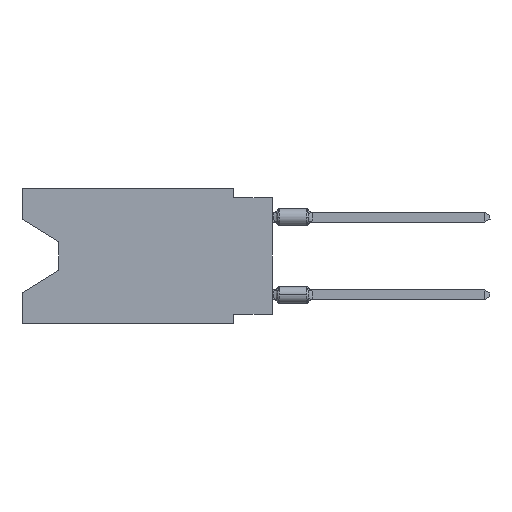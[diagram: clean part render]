
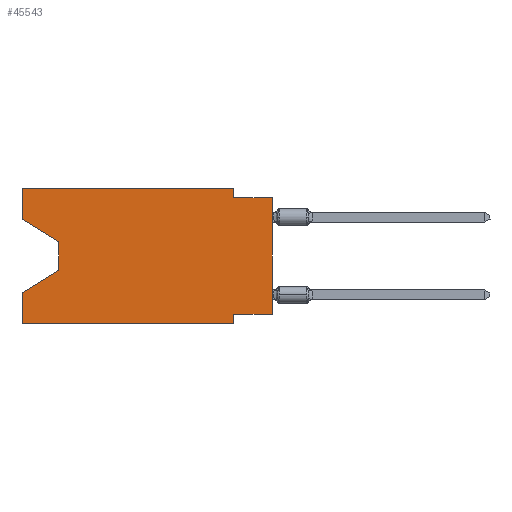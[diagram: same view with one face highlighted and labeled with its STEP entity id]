
A CAD part, left-side view. The second image highlights one B-rep face of the part: STEP entity #45543.
In plain terms, the highlighted planar face has unit normal (-1, 0, 0).
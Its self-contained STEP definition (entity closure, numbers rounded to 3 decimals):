
#326 = ORIENTED_EDGE ( 'NONE', *, *, #33293, .T. ) ;
#357 = DIRECTION ( 'NONE',  ( 0., -1., 0. ) ) ;
#640 = VECTOR ( 'NONE', #40639, 1000. ) ;
#901 = DIRECTION ( 'NONE',  ( 0., 0., -1. ) ) ;
#928 = EDGE_CURVE ( 'NONE', #18236, #33022, #54959, .T. ) ;
#1492 = CARTESIAN_POINT ( 'NONE',  ( 0., 0., -0.635 ) ) ;
#1679 = CARTESIAN_POINT ( 'NONE',  ( 0., 16.383, 0. ) ) ;
#2048 = VECTOR ( 'NONE', #901, 1000. ) ;
#2171 = LINE ( 'NONE', #29667, #26719 ) ;
#2493 = LINE ( 'NONE', #36974, #19120 ) ;
#5666 = CARTESIAN_POINT ( 'NONE',  ( 0., 13.97, -5.385 ) ) ;
#6044 = CARTESIAN_POINT ( 'NONE',  ( 0., 2.54, -8.89 ) ) ;
#7117 = LINE ( 'NONE', #29249, #27710 ) ;
#7543 = EDGE_CURVE ( 'NONE', #15446, #8250, #2493, .T. ) ;
#7650 = CARTESIAN_POINT ( 'NONE',  ( 0., 13.97, -3.505 ) ) ;
#8250 = VERTEX_POINT ( 'NONE', #22980 ) ;
#8898 = DIRECTION ( 'NONE',  ( 1., 0., 0. ) ) ;
#10454 = CARTESIAN_POINT ( 'NONE',  ( 0., 0., -8.255 ) ) ;
#10478 = ORIENTED_EDGE ( 'NONE', *, *, #29327, .T. ) ;
#11455 = LINE ( 'NONE', #28986, #30666 ) ;
#13536 = AXIS2_PLACEMENT_3D ( 'NONE', #30455, #8898, #48000 ) ;
#13838 = VERTEX_POINT ( 'NONE', #42373 ) ;
#15159 = DIRECTION ( 'NONE',  ( 0., 0., -1. ) ) ;
#15446 = VERTEX_POINT ( 'NONE', #5666 ) ;
#15514 = LINE ( 'NONE', #1492, #50405 ) ;
#17047 = CARTESIAN_POINT ( 'NONE',  ( 0., 16.383, -2.038 ) ) ;
#18236 = VERTEX_POINT ( 'NONE', #27883 ) ;
#19120 = VECTOR ( 'NONE', #33236, 1000. ) ;
#20636 = ORIENTED_EDGE ( 'NONE', *, *, #44938, .F. ) ;
#21025 = DIRECTION ( 'NONE',  ( 0., -1., 0. ) ) ;
#21209 = EDGE_CURVE ( 'NONE', #27404, #33022, #15514, .T. ) ;
#21676 = ORIENTED_EDGE ( 'NONE', *, *, #928, .T. ) ;
#22693 = VERTEX_POINT ( 'NONE', #22965 ) ;
#22965 = CARTESIAN_POINT ( 'NONE',  ( 0., 16.383, 0. ) ) ;
#22980 = CARTESIAN_POINT ( 'NONE',  ( 0., 16.383, -6.852 ) ) ;
#23207 = DIRECTION ( 'NONE',  ( 0., 0., 1. ) ) ;
#23216 = VECTOR ( 'NONE', #37845, 1000. ) ;
#24538 = CARTESIAN_POINT ( 'NONE',  ( 0., 2.54, 0. ) ) ;
#24879 = VERTEX_POINT ( 'NONE', #24538 ) ;
#26423 = PLANE ( 'NONE',  #13536 ) ;
#26498 = LINE ( 'NONE', #35976, #47825 ) ;
#26719 = VECTOR ( 'NONE', #21025, 1000. ) ;
#27404 = VERTEX_POINT ( 'NONE', #27721 ) ;
#27682 = CARTESIAN_POINT ( 'NONE',  ( 0., 2.54, -8.255 ) ) ;
#27710 = VECTOR ( 'NONE', #15159, 1000. ) ;
#27721 = CARTESIAN_POINT ( 'NONE',  ( 0., 2.54, -0.635 ) ) ;
#27883 = CARTESIAN_POINT ( 'NONE',  ( 0., 0., -8.255 ) ) ;
#28986 = CARTESIAN_POINT ( 'NONE',  ( 0., 16.383, -2.038 ) ) ;
#29249 = CARTESIAN_POINT ( 'NONE',  ( 0., 2.54, 0. ) ) ;
#29327 = EDGE_CURVE ( 'NONE', #54973, #13838, #2171, .T. ) ;
#29667 = CARTESIAN_POINT ( 'NONE',  ( 0., 16.383, -8.89 ) ) ;
#30136 = EDGE_CURVE ( 'NONE', #24879, #27404, #7117, .T. ) ;
#30376 = EDGE_CURVE ( 'NONE', #56284, #13838, #40248, .T. ) ;
#30455 = CARTESIAN_POINT ( 'NONE',  ( 0., 16.383, 0. ) ) ;
#30666 = VECTOR ( 'NONE', #42218, 1000. ) ;
#31108 = ORIENTED_EDGE ( 'NONE', *, *, #53416, .T. ) ;
#32313 = VERTEX_POINT ( 'NONE', #17047 ) ;
#33022 = VERTEX_POINT ( 'NONE', #52822 ) ;
#33117 = CARTESIAN_POINT ( 'NONE',  ( 0., 0., 0. ) ) ;
#33236 = DIRECTION ( 'NONE',  ( 0., 0.855, -0.519 ) ) ;
#33293 = EDGE_CURVE ( 'NONE', #36830, #15446, #47032, .T. ) ;
#34104 = ORIENTED_EDGE ( 'NONE', *, *, #7543, .T. ) ;
#34404 = ORIENTED_EDGE ( 'NONE', *, *, #30376, .F. ) ;
#34439 = ORIENTED_EDGE ( 'NONE', *, *, #36665, .F. ) ;
#35976 = CARTESIAN_POINT ( 'NONE',  ( 0., 16.383, 0. ) ) ;
#36601 = LINE ( 'NONE', #10454, #640 ) ;
#36665 = EDGE_CURVE ( 'NONE', #22693, #24879, #26498, .T. ) ;
#36668 = VECTOR ( 'NONE', #42919, 1000. ) ;
#36830 = VERTEX_POINT ( 'NONE', #41702 ) ;
#36974 = CARTESIAN_POINT ( 'NONE',  ( 0., 13.97, -5.385 ) ) ;
#37442 = ORIENTED_EDGE ( 'NONE', *, *, #46718, .F. ) ;
#37845 = DIRECTION ( 'NONE',  ( 0., 0., -1. ) ) ;
#39889 = EDGE_CURVE ( 'NONE', #54973, #8250, #46961, .T. ) ;
#40248 = LINE ( 'NONE', #6044, #2048 ) ;
#40639 = DIRECTION ( 'NONE',  ( 0., 1., 0. ) ) ;
#41037 = LINE ( 'NONE', #1679, #41164 ) ;
#41115 = DIRECTION ( 'NONE',  ( 0., -1., 0. ) ) ;
#41164 = VECTOR ( 'NONE', #23207, 1000. ) ;
#41702 = CARTESIAN_POINT ( 'NONE',  ( 0., 13.97, -3.505 ) ) ;
#42218 = DIRECTION ( 'NONE',  ( 0., -0.855, -0.519 ) ) ;
#42219 = ORIENTED_EDGE ( 'NONE', *, *, #21209, .F. ) ;
#42373 = CARTESIAN_POINT ( 'NONE',  ( 0., 2.54, -8.89 ) ) ;
#42919 = DIRECTION ( 'NONE',  ( 0., 0., 1. ) ) ;
#43402 = FACE_OUTER_BOUND ( 'NONE', #47836, .T. ) ;
#44938 = EDGE_CURVE ( 'NONE', #18236, #56284, #36601, .T. ) ;
#45543 = ADVANCED_FACE ( 'NONE', ( #43402 ), #26423, .F. ) ;
#46339 = DIRECTION ( 'NONE',  ( 0., 0., 1. ) ) ;
#46718 = EDGE_CURVE ( 'NONE', #32313, #22693, #41037, .T. ) ;
#46961 = LINE ( 'NONE', #55311, #36668 ) ;
#47032 = LINE ( 'NONE', #7650, #23216 ) ;
#47825 = VECTOR ( 'NONE', #357, 1000. ) ;
#47836 = EDGE_LOOP ( 'NONE', ( #31108, #326, #34104, #56124, #10478, #34404, #20636, #21676, #42219, #48486, #34439, #37442 ) ) ;
#48000 = DIRECTION ( 'NONE',  ( 0., 0., -1. ) ) ;
#48486 = ORIENTED_EDGE ( 'NONE', *, *, #30136, .F. ) ;
#50405 = VECTOR ( 'NONE', #41115, 1000. ) ;
#51824 = VECTOR ( 'NONE', #46339, 1000. ) ;
#52822 = CARTESIAN_POINT ( 'NONE',  ( 0., 0., -0.635 ) ) ;
#53416 = EDGE_CURVE ( 'NONE', #32313, #36830, #11455, .T. ) ;
#54959 = LINE ( 'NONE', #33117, #51824 ) ;
#54973 = VERTEX_POINT ( 'NONE', #56723 ) ;
#55311 = CARTESIAN_POINT ( 'NONE',  ( 0., 16.383, 0. ) ) ;
#56124 = ORIENTED_EDGE ( 'NONE', *, *, #39889, .F. ) ;
#56284 = VERTEX_POINT ( 'NONE', #27682 ) ;
#56723 = CARTESIAN_POINT ( 'NONE',  ( 0., 16.383, -8.89 ) ) ;
